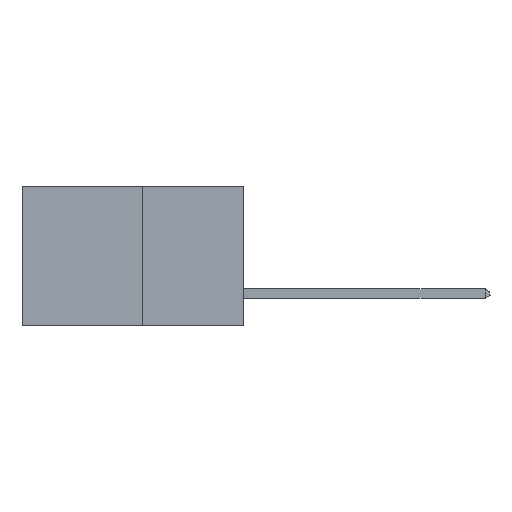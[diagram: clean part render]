
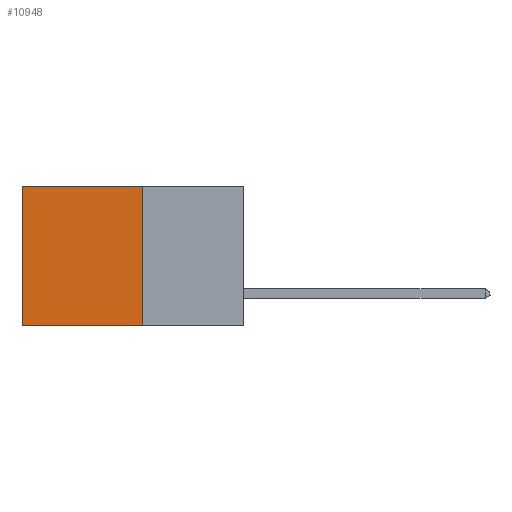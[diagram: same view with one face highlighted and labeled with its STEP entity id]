
A CAD part, left-side view. The second image highlights one B-rep face of the part: STEP entity #10948.
In plain terms, the highlighted planar face has unit normal (-1, 0, 0).
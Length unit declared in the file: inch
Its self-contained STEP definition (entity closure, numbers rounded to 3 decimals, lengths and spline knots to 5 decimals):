
#93 = EDGE_CURVE ( 'NONE', #1149, #741, #7866, .T. ) ;
#104 = CARTESIAN_POINT ( 'NONE',  ( 0.277, 0.59, -0.37 ) ) ;
#134 = EDGE_CURVE ( 'NONE', #9671, #6471, #6392, .T. ) ;
#395 = EDGE_CURVE ( 'NONE', #6471, #741, #11935, .T. ) ;
#504 = ORIENTED_EDGE ( 'NONE', *, *, #395, .T. ) ;
#570 = AXIS2_PLACEMENT_3D ( 'NONE', #8239, #4320, #11171 ) ;
#741 = VERTEX_POINT ( 'NONE', #5569 ) ;
#795 = VECTOR ( 'NONE', #7514, 39.37008 ) ;
#1149 = VERTEX_POINT ( 'NONE', #6615 ) ;
#1205 = EDGE_CURVE ( 'NONE', #9671, #1149, #8119, .T. ) ;
#1700 = ORIENTED_EDGE ( 'NONE', *, *, #1205, .F. ) ;
#1718 = CARTESIAN_POINT ( 'NONE',  ( 0.277, 0.27, 0. ) ) ;
#2174 = VECTOR ( 'NONE', #11643, 39.37008 ) ;
#3571 = VECTOR ( 'NONE', #9204, 39.37008 ) ;
#4015 = ORIENTED_EDGE ( 'NONE', *, *, #134, .T. ) ;
#4320 = DIRECTION ( 'NONE',  ( 1., 0., 0. ) ) ;
#5569 = CARTESIAN_POINT ( 'NONE',  ( 0.277, 0.59, -0.37 ) ) ;
#6392 = LINE ( 'NONE', #11609, #3571 ) ;
#6471 = VERTEX_POINT ( 'NONE', #12697 ) ;
#6615 = CARTESIAN_POINT ( 'NONE',  ( 0.277, 0.27, -0.37 ) ) ;
#7514 = DIRECTION ( 'NONE',  ( 0., 0., -1. ) ) ;
#7590 = ORIENTED_EDGE ( 'NONE', *, *, #93, .F. ) ;
#7866 = LINE ( 'NONE', #12316, #12386 ) ;
#8119 = LINE ( 'NONE', #8409, #2174 ) ;
#8239 = CARTESIAN_POINT ( 'NONE',  ( 0.277, 0.27, -0.37 ) ) ;
#8409 = CARTESIAN_POINT ( 'NONE',  ( 0.277, 0.27, -0.37 ) ) ;
#9204 = DIRECTION ( 'NONE',  ( 0., 1., 0. ) ) ;
#9671 = VERTEX_POINT ( 'NONE', #1718 ) ;
#10203 = PLANE ( 'NONE',  #570 ) ;
#10404 = DIRECTION ( 'NONE',  ( 0., 1., 0. ) ) ;
#10948 = ADVANCED_FACE ( 'NONE', ( #11650 ), #10203, .F. ) ;
#11171 = DIRECTION ( 'NONE',  ( 0., 0., -1. ) ) ;
#11609 = CARTESIAN_POINT ( 'NONE',  ( 0.277, 0.27, 0. ) ) ;
#11643 = DIRECTION ( 'NONE',  ( 0., 0., -1. ) ) ;
#11650 = FACE_OUTER_BOUND ( 'NONE', #12400, .T. ) ;
#11935 = LINE ( 'NONE', #104, #795 ) ;
#12316 = CARTESIAN_POINT ( 'NONE',  ( 0.277, 0.27, -0.37 ) ) ;
#12386 = VECTOR ( 'NONE', #10404, 39.37008 ) ;
#12400 = EDGE_LOOP ( 'NONE', ( #504, #7590, #1700, #4015 ) ) ;
#12697 = CARTESIAN_POINT ( 'NONE',  ( 0.277, 0.59, 0. ) ) ;
